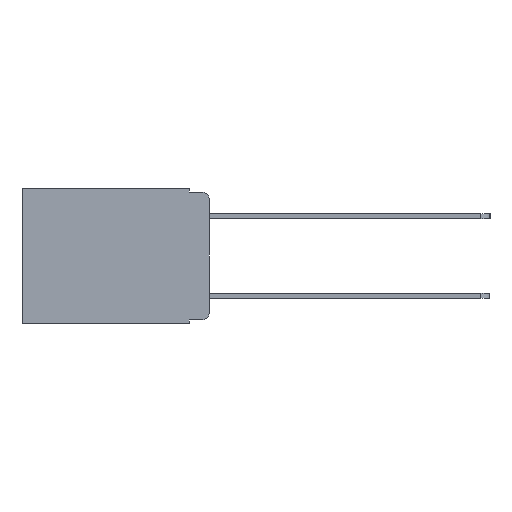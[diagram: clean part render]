
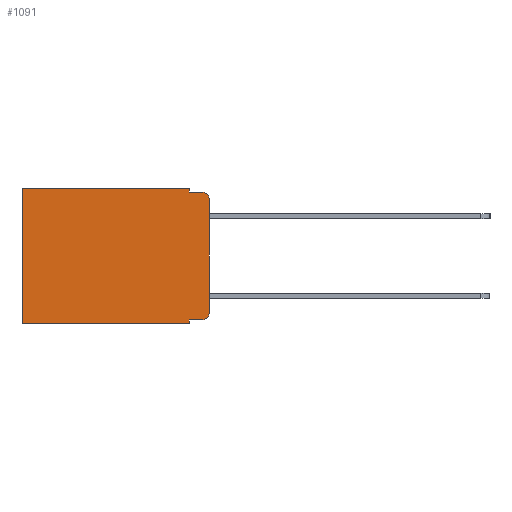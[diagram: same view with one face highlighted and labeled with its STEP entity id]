
A CAD part, left-side view. The second image highlights one B-rep face of the part: STEP entity #1091.
In plain terms, the highlighted planar face has unit normal (-1, 0, 0).
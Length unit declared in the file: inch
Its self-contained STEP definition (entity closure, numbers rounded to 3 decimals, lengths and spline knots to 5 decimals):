
#149 = CARTESIAN_POINT ( 'NONE',  ( 0.298, 0.051, -0.343 ) ) ;
#906 = LINE ( 'NONE', #9154, #17303 ) ;
#1000 = ORIENTED_EDGE ( 'NONE', *, *, #15413, .F. ) ;
#1061 = CARTESIAN_POINT ( 'NONE',  ( 0.298, 0.473, -0.343 ) ) ;
#1091 = ADVANCED_FACE ( 'NONE', ( #5306 ), #19728, .F. ) ;
#1135 = VECTOR ( 'NONE', #17856, 39.37008 ) ;
#1522 = VECTOR ( 'NONE', #18560, 39.37008 ) ;
#1634 = ORIENTED_EDGE ( 'NONE', *, *, #16309, .T. ) ;
#1680 = CARTESIAN_POINT ( 'NONE',  ( 0.298, 0.473, 0. ) ) ;
#1858 = VECTOR ( 'NONE', #16624, 39.37008 ) ;
#1904 = EDGE_CURVE ( 'NONE', #20055, #7644, #6964, .T. ) ;
#1965 = CARTESIAN_POINT ( 'NONE',  ( 0.298, 0.02, -0.333 ) ) ;
#2633 = DIRECTION ( 'NONE',  ( 0., -1., 0. ) ) ;
#2685 = ORIENTED_EDGE ( 'NONE', *, *, #1904, .F. ) ;
#2816 = CARTESIAN_POINT ( 'NONE',  ( 0.298, 0.051, -0.333 ) ) ;
#2883 = CARTESIAN_POINT ( 'NONE',  ( 0.298, 0.02, -0.03 ) ) ;
#3104 = CIRCLE ( 'NONE', #18711, 0.02 ) ;
#3373 = VERTEX_POINT ( 'NONE', #1965 ) ;
#3741 = ORIENTED_EDGE ( 'NONE', *, *, #11340, .T. ) ;
#3766 = ORIENTED_EDGE ( 'NONE', *, *, #16418, .F. ) ;
#3845 = VERTEX_POINT ( 'NONE', #1680 ) ;
#4637 = DIRECTION ( 'NONE',  ( 0., 0., -1. ) ) ;
#4928 = VERTEX_POINT ( 'NONE', #18951 ) ;
#5059 = LINE ( 'NONE', #17860, #13830 ) ;
#5126 = CARTESIAN_POINT ( 'NONE',  ( 0.298, 0.02, -0.313 ) ) ;
#5306 = FACE_OUTER_BOUND ( 'NONE', #10158, .T. ) ;
#6561 = LINE ( 'NONE', #10462, #14360 ) ;
#6597 = DIRECTION ( 'NONE',  ( 0., 0., -1. ) ) ;
#6713 = DIRECTION ( 'NONE',  ( 0., 0., -1. ) ) ;
#6872 = VERTEX_POINT ( 'NONE', #9504 ) ;
#6964 = LINE ( 'NONE', #18581, #1522 ) ;
#7063 = CARTESIAN_POINT ( 'NONE',  ( 0.298, 0.051, -0.01 ) ) ;
#7644 = VERTEX_POINT ( 'NONE', #1061 ) ;
#8205 = LINE ( 'NONE', #15852, #16355 ) ;
#9154 = CARTESIAN_POINT ( 'NONE',  ( 0.298, 0.051, -0.333 ) ) ;
#9445 = VERTEX_POINT ( 'NONE', #18160 ) ;
#9504 = CARTESIAN_POINT ( 'NONE',  ( 0.298, 0.02, -0.01 ) ) ;
#10022 = LINE ( 'NONE', #10738, #17083 ) ;
#10158 = EDGE_LOOP ( 'NONE', ( #15313, #19227, #3766, #1000, #1634, #14364, #2685, #15758, #19673, #3741 ) ) ;
#10373 = DIRECTION ( 'NONE',  ( 0., 0., -1. ) ) ;
#10423 = CARTESIAN_POINT ( 'NONE',  ( 0.298, 0.051, 0. ) ) ;
#10462 = CARTESIAN_POINT ( 'NONE',  ( 0.298, 0.473, 0. ) ) ;
#10555 = CARTESIAN_POINT ( 'NONE',  ( 0.298, 0., 0. ) ) ;
#10640 = DIRECTION ( 'NONE',  ( 0., 0., -1. ) ) ;
#10738 = CARTESIAN_POINT ( 'NONE',  ( 0.298, 0.051, -0.01 ) ) ;
#10891 = VERTEX_POINT ( 'NONE', #2816 ) ;
#11340 = EDGE_CURVE ( 'NONE', #3373, #4928, #15726, .T. ) ;
#12328 = EDGE_CURVE ( 'NONE', #10891, #3373, #906, .T. ) ;
#13370 = EDGE_CURVE ( 'NONE', #10891, #20055, #8205, .T. ) ;
#13437 = AXIS2_PLACEMENT_3D ( 'NONE', #16219, #18829, #10640 ) ;
#13467 = AXIS2_PLACEMENT_3D ( 'NONE', #5126, #15962, #6713 ) ;
#13479 = LINE ( 'NONE', #16387, #1135 ) ;
#13830 = VECTOR ( 'NONE', #10373, 39.37008 ) ;
#13994 = DIRECTION ( 'NONE',  ( -1., 0., 0. ) ) ;
#14360 = VECTOR ( 'NONE', #19421, 39.37008 ) ;
#14364 = ORIENTED_EDGE ( 'NONE', *, *, #14431, .T. ) ;
#14431 = EDGE_CURVE ( 'NONE', #3845, #7644, #6561, .T. ) ;
#15313 = ORIENTED_EDGE ( 'NONE', *, *, #19368, .F. ) ;
#15413 = EDGE_CURVE ( 'NONE', #16199, #16112, #5059, .T. ) ;
#15726 = CIRCLE ( 'NONE', #13467, 0.02 ) ;
#15758 = ORIENTED_EDGE ( 'NONE', *, *, #13370, .F. ) ;
#15852 = CARTESIAN_POINT ( 'NONE',  ( 0.298, 0.051, 0. ) ) ;
#15962 = DIRECTION ( 'NONE',  ( -1., 0., 0. ) ) ;
#16112 = VERTEX_POINT ( 'NONE', #7063 ) ;
#16199 = VERTEX_POINT ( 'NONE', #10423 ) ;
#16219 = CARTESIAN_POINT ( 'NONE',  ( 0.298, 0., 0. ) ) ;
#16309 = EDGE_CURVE ( 'NONE', #16199, #3845, #18932, .T. ) ;
#16355 = VECTOR ( 'NONE', #6597, 39.37008 ) ;
#16387 = CARTESIAN_POINT ( 'NONE',  ( 0.298, 0., 0. ) ) ;
#16418 = EDGE_CURVE ( 'NONE', #16112, #6872, #10022, .T. ) ;
#16624 = DIRECTION ( 'NONE',  ( 0., 1., 0. ) ) ;
#17083 = VECTOR ( 'NONE', #18226, 39.37008 ) ;
#17303 = VECTOR ( 'NONE', #2633, 39.37008 ) ;
#17408 = EDGE_CURVE ( 'NONE', #9445, #6872, #3104, .T. ) ;
#17856 = DIRECTION ( 'NONE',  ( 0., 0., -1. ) ) ;
#17860 = CARTESIAN_POINT ( 'NONE',  ( 0.298, 0.051, 0. ) ) ;
#18160 = CARTESIAN_POINT ( 'NONE',  ( 0.298, 0., -0.03 ) ) ;
#18226 = DIRECTION ( 'NONE',  ( 0., -1., 0. ) ) ;
#18560 = DIRECTION ( 'NONE',  ( 0., 1., 0. ) ) ;
#18581 = CARTESIAN_POINT ( 'NONE',  ( 0.298, 0., -0.343 ) ) ;
#18711 = AXIS2_PLACEMENT_3D ( 'NONE', #2883, #13994, #4637 ) ;
#18829 = DIRECTION ( 'NONE',  ( 1., 0., 0. ) ) ;
#18932 = LINE ( 'NONE', #10555, #1858 ) ;
#18951 = CARTESIAN_POINT ( 'NONE',  ( 0.298, 0., -0.313 ) ) ;
#19227 = ORIENTED_EDGE ( 'NONE', *, *, #17408, .T. ) ;
#19368 = EDGE_CURVE ( 'NONE', #9445, #4928, #13479, .T. ) ;
#19421 = DIRECTION ( 'NONE',  ( 0., 0., -1. ) ) ;
#19673 = ORIENTED_EDGE ( 'NONE', *, *, #12328, .T. ) ;
#19728 = PLANE ( 'NONE',  #13437 ) ;
#20055 = VERTEX_POINT ( 'NONE', #149 ) ;
